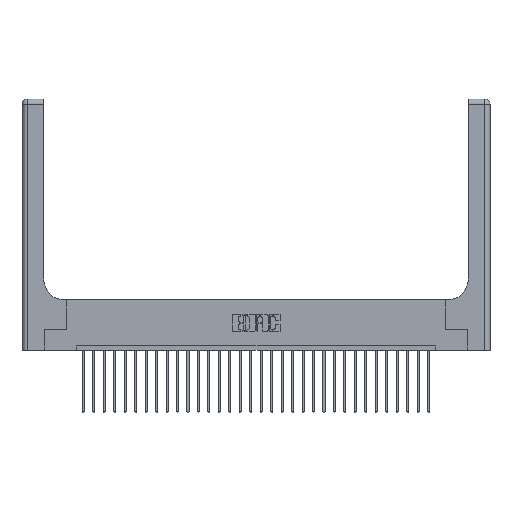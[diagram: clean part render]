
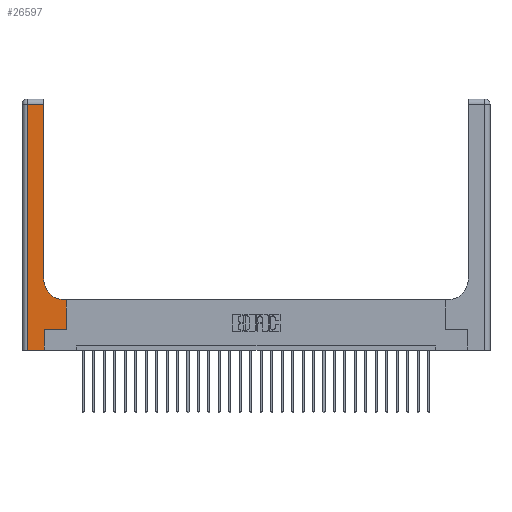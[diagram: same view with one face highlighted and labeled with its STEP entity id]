
A CAD part, top view. The second image highlights one B-rep face of the part: STEP entity #26597.
In plain terms, the highlighted planar face has unit normal (0, 0, 1).
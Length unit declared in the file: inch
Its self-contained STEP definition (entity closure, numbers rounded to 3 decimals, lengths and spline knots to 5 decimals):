
#213 = AXIS2_PLACEMENT_3D ( 'NONE', #15762, #3056, #17793 ) ;
#646 = LINE ( 'NONE', #25820, #27102 ) ;
#1230 = EDGE_LOOP ( 'NONE', ( #23101, #24600, #1468, #19607, #6960, #11319, #7422, #24560, #2112 ) ) ;
#1468 = ORIENTED_EDGE ( 'NONE', *, *, #7981, .T. ) ;
#1699 = AXIS2_PLACEMENT_3D ( 'NONE', #17661, #21840, #5130 ) ;
#1853 = EDGE_CURVE ( 'NONE', #9176, #27177, #24871, .T. ) ;
#2112 = ORIENTED_EDGE ( 'NONE', *, *, #1853, .T. ) ;
#2452 = DIRECTION ( 'NONE',  ( 1., 0., 0. ) ) ;
#2575 = EDGE_CURVE ( 'NONE', #4023, #4485, #8288, .T. ) ;
#3053 = VECTOR ( 'NONE', #25463, 39.37008 ) ;
#3056 = DIRECTION ( 'NONE',  ( 0., 0., -1. ) ) ;
#3287 = DIRECTION ( 'NONE',  ( -1., 0., 0. ) ) ;
#3453 = CARTESIAN_POINT ( 'NONE',  ( 0.528, 0.25, 0.37 ) ) ;
#4023 = VERTEX_POINT ( 'NONE', #22755 ) ;
#4204 = DIRECTION ( 'NONE',  ( 1., 0., 0. ) ) ;
#4302 = CARTESIAN_POINT ( 'NONE',  ( 0.26, 3., 0.37 ) ) ;
#4375 = CARTESIAN_POINT ( 'NONE',  ( 0., 2.94, 0.37 ) ) ;
#4387 = CARTESIAN_POINT ( 'NONE',  ( 0.265, 0.25, 0.37 ) ) ;
#4485 = VERTEX_POINT ( 'NONE', #3453 ) ;
#4654 = VECTOR ( 'NONE', #4204, 39.37008 ) ;
#5130 = DIRECTION ( 'NONE',  ( -1., 0., 0. ) ) ;
#6050 = EDGE_CURVE ( 'NONE', #10205, #4023, #16686, .T. ) ;
#6222 = CARTESIAN_POINT ( 'NONE',  ( 0.06, 3., 0.37 ) ) ;
#6266 = DIRECTION ( 'NONE',  ( 0., 1., 0. ) ) ;
#6317 = DIRECTION ( 'NONE',  ( 0., -1., 0. ) ) ;
#6519 = EDGE_CURVE ( 'NONE', #15934, #9176, #8116, .T. ) ;
#6960 = ORIENTED_EDGE ( 'NONE', *, *, #6050, .T. ) ;
#7354 = PLANE ( 'NONE',  #1699 ) ;
#7420 = CARTESIAN_POINT ( 'NONE',  ( 0.26, 0.85, 0.37 ) ) ;
#7422 = ORIENTED_EDGE ( 'NONE', *, *, #24397, .T. ) ;
#7551 = CARTESIAN_POINT ( 'NONE',  ( 0.51, 0.6, 0.37 ) ) ;
#7981 = EDGE_CURVE ( 'NONE', #27110, #19376, #14610, .T. ) ;
#8116 = LINE ( 'NONE', #26588, #11067 ) ;
#8288 = LINE ( 'NONE', #4387, #4654 ) ;
#8996 = VECTOR ( 'NONE', #6317, 39.37008 ) ;
#9147 = LINE ( 'NONE', #4375, #17707 ) ;
#9176 = VERTEX_POINT ( 'NONE', #7551 ) ;
#9252 = CARTESIAN_POINT ( 'NONE',  ( 0.06, 2.94, 0.37 ) ) ;
#9889 = EDGE_CURVE ( 'NONE', #19376, #10205, #646, .T. ) ;
#10205 = VERTEX_POINT ( 'NONE', #24122 ) ;
#10736 = CARTESIAN_POINT ( 'NONE',  ( 0.528, 0.25, 0.37 ) ) ;
#10767 = CARTESIAN_POINT ( 'NONE',  ( 0.265, 0., 0.37 ) ) ;
#11067 = VECTOR ( 'NONE', #3287, 39.37008 ) ;
#11319 = ORIENTED_EDGE ( 'NONE', *, *, #2575, .T. ) ;
#12071 = VECTOR ( 'NONE', #6266, 39.37008 ) ;
#14610 = LINE ( 'NONE', #6222, #8996 ) ;
#15404 = LINE ( 'NONE', #10736, #24041 ) ;
#15517 = CARTESIAN_POINT ( 'NONE',  ( 0.528, 0.6, 0.37 ) ) ;
#15762 = CARTESIAN_POINT ( 'NONE',  ( 0.51, 0.85, 0.37 ) ) ;
#15934 = VERTEX_POINT ( 'NONE', #15517 ) ;
#16686 = LINE ( 'NONE', #10767, #12071 ) ;
#17661 = CARTESIAN_POINT ( 'NONE',  ( 0., 3., 0.37 ) ) ;
#17707 = VECTOR ( 'NONE', #23330, 39.37008 ) ;
#17793 = DIRECTION ( 'NONE',  ( 1., 0., 0. ) ) ;
#19376 = VERTEX_POINT ( 'NONE', #23103 ) ;
#19607 = ORIENTED_EDGE ( 'NONE', *, *, #9889, .T. ) ;
#20972 = FACE_OUTER_BOUND ( 'NONE', #1230, .T. ) ;
#21135 = EDGE_CURVE ( 'NONE', #27177, #26663, #25537, .T. ) ;
#21840 = DIRECTION ( 'NONE',  ( 0., 0., -1. ) ) ;
#22755 = CARTESIAN_POINT ( 'NONE',  ( 0.265, 0.25, 0.37 ) ) ;
#23101 = ORIENTED_EDGE ( 'NONE', *, *, #21135, .T. ) ;
#23103 = CARTESIAN_POINT ( 'NONE',  ( 0.06, 0., 0.37 ) ) ;
#23330 = DIRECTION ( 'NONE',  ( -1., 0., 0. ) ) ;
#24041 = VECTOR ( 'NONE', #25532, 39.37008 ) ;
#24122 = CARTESIAN_POINT ( 'NONE',  ( 0.265, 0., 0.37 ) ) ;
#24359 = EDGE_CURVE ( 'NONE', #26663, #27110, #9147, .T. ) ;
#24397 = EDGE_CURVE ( 'NONE', #4485, #15934, #15404, .T. ) ;
#24560 = ORIENTED_EDGE ( 'NONE', *, *, #6519, .T. ) ;
#24600 = ORIENTED_EDGE ( 'NONE', *, *, #24359, .T. ) ;
#24871 = CIRCLE ( 'NONE', #213, 0.25 ) ;
#25463 = DIRECTION ( 'NONE',  ( 0., 1., 0. ) ) ;
#25532 = DIRECTION ( 'NONE',  ( 0., 1., 0. ) ) ;
#25537 = LINE ( 'NONE', #4302, #3053 ) ;
#25820 = CARTESIAN_POINT ( 'NONE',  ( 0., 0., 0.37 ) ) ;
#26301 = CARTESIAN_POINT ( 'NONE',  ( 0.26, 2.94, 0.37 ) ) ;
#26588 = CARTESIAN_POINT ( 'NONE',  ( 0.26, 0.6, 0.37 ) ) ;
#26597 = ADVANCED_FACE ( 'NONE', ( #20972 ), #7354, .F. ) ;
#26663 = VERTEX_POINT ( 'NONE', #26301 ) ;
#27102 = VECTOR ( 'NONE', #2452, 39.37008 ) ;
#27110 = VERTEX_POINT ( 'NONE', #9252 ) ;
#27177 = VERTEX_POINT ( 'NONE', #7420 ) ;
